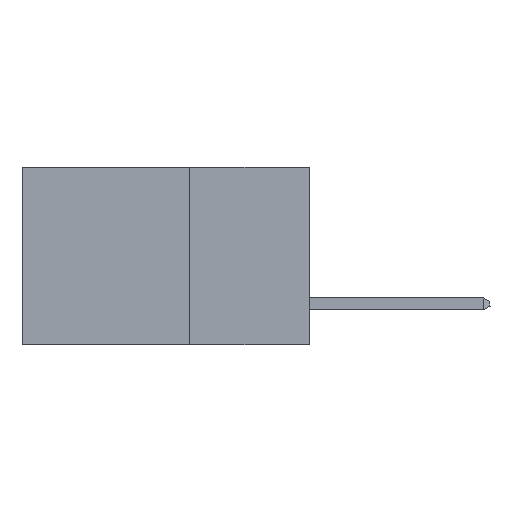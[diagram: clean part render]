
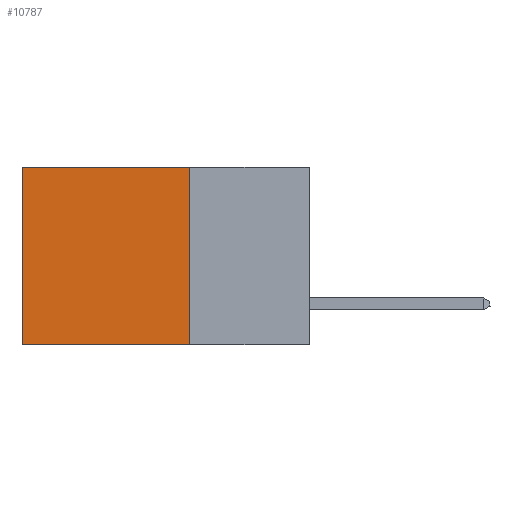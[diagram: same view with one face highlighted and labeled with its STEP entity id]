
A CAD part, left-side view. The second image highlights one B-rep face of the part: STEP entity #10787.
In plain terms, the highlighted planar face has unit normal (-1, 0, 0).
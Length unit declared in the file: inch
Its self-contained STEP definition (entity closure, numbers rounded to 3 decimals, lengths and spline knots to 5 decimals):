
#254 = ORIENTED_EDGE ( 'NONE', *, *, #13384, .F. ) ;
#640 = ORIENTED_EDGE ( 'NONE', *, *, #11961, .T. ) ;
#1582 = CARTESIAN_POINT ( 'NONE',  ( 0.2875, 0.25, 0. ) ) ;
#2055 = LINE ( 'NONE', #4404, #6920 ) ;
#2199 = ORIENTED_EDGE ( 'NONE', *, *, #7461, .T. ) ;
#2424 = ORIENTED_EDGE ( 'NONE', *, *, #17418, .F. ) ;
#3106 = CARTESIAN_POINT ( 'NONE',  ( 0.2875, 0.25, -0.37 ) ) ;
#3911 = CARTESIAN_POINT ( 'NONE',  ( 0.2875, 0.25, 0. ) ) ;
#4404 = CARTESIAN_POINT ( 'NONE',  ( 0.2875, 0.25, 0. ) ) ;
#4754 = LINE ( 'NONE', #5769, #14977 ) ;
#5399 = CARTESIAN_POINT ( 'NONE',  ( 0.2875, 0.6, 0. ) ) ;
#5542 = VERTEX_POINT ( 'NONE', #1582 ) ;
#5566 = LINE ( 'NONE', #9293, #20317 ) ;
#5769 = CARTESIAN_POINT ( 'NONE',  ( 0.2875, 0.25, -0.37 ) ) ;
#6504 = VERTEX_POINT ( 'NONE', #3106 ) ;
#6920 = VECTOR ( 'NONE', #11522, 39.37008 ) ;
#7461 = EDGE_CURVE ( 'NONE', #5542, #19331, #2055, .T. ) ;
#9222 = DIRECTION ( 'NONE',  ( 0., 0., -1. ) ) ;
#9293 = CARTESIAN_POINT ( 'NONE',  ( 0.2875, 0.25, 0. ) ) ;
#10001 = DIRECTION ( 'NONE',  ( 1., 0., 0. ) ) ;
#10787 = ADVANCED_FACE ( 'NONE', ( #18621 ), #11270, .F. ) ;
#11270 = PLANE ( 'NONE',  #16066 ) ;
#11458 = VECTOR ( 'NONE', #18290, 39.37008 ) ;
#11522 = DIRECTION ( 'NONE',  ( 0., 1., 0. ) ) ;
#11961 = EDGE_CURVE ( 'NONE', #19331, #14969, #19066, .T. ) ;
#12919 = EDGE_LOOP ( 'NONE', ( #640, #2424, #254, #2199 ) ) ;
#13384 = EDGE_CURVE ( 'NONE', #5542, #6504, #5566, .T. ) ;
#14969 = VERTEX_POINT ( 'NONE', #20934 ) ;
#14977 = VECTOR ( 'NONE', #17376, 39.37008 ) ;
#16066 = AXIS2_PLACEMENT_3D ( 'NONE', #3911, #10001, #16401 ) ;
#16401 = DIRECTION ( 'NONE',  ( 0., 0., -1. ) ) ;
#16872 = CARTESIAN_POINT ( 'NONE',  ( 0.2875, 0.6, 0. ) ) ;
#17376 = DIRECTION ( 'NONE',  ( 0., 1., 0. ) ) ;
#17418 = EDGE_CURVE ( 'NONE', #6504, #14969, #4754, .T. ) ;
#18290 = DIRECTION ( 'NONE',  ( 0., 0., -1. ) ) ;
#18621 = FACE_OUTER_BOUND ( 'NONE', #12919, .T. ) ;
#19066 = LINE ( 'NONE', #16872, #11458 ) ;
#19331 = VERTEX_POINT ( 'NONE', #5399 ) ;
#20317 = VECTOR ( 'NONE', #9222, 39.37008 ) ;
#20934 = CARTESIAN_POINT ( 'NONE',  ( 0.2875, 0.6, -0.37 ) ) ;
